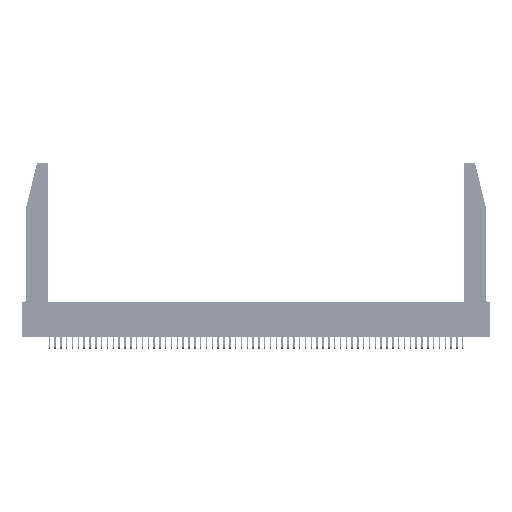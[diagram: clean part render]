
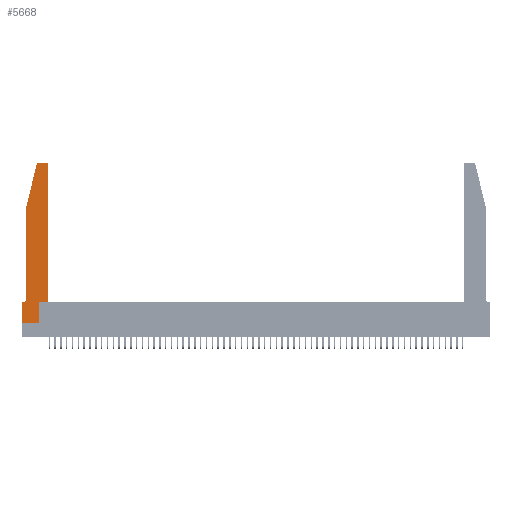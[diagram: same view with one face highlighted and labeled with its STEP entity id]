
A CAD part, top view. The second image highlights one B-rep face of the part: STEP entity #5668.
In plain terms, the highlighted planar face has unit normal (0, 0, 1).
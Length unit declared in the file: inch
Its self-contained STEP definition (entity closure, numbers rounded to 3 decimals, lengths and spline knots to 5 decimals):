
#886 = LINE ( 'NONE', #34064, #15802 ) ;
#995 = DIRECTION ( 'NONE',  ( 1., 0., 0. ) ) ;
#1114 = DIRECTION ( 'NONE',  ( 1., 0., 0. ) ) ;
#1176 = ORIENTED_EDGE ( 'NONE', *, *, #48175, .T. ) ;
#2003 = VECTOR ( 'NONE', #14188, 39.37008 ) ;
#2604 = AXIS2_PLACEMENT_3D ( 'NONE', #47285, #15888, #20061 ) ;
#2913 = CARTESIAN_POINT ( 'NONE',  ( 0.284, 2.75, 0.37 ) ) ;
#3391 = VERTEX_POINT ( 'NONE', #58541 ) ;
#3454 = VERTEX_POINT ( 'NONE', #50158 ) ;
#3979 = ORIENTED_EDGE ( 'NONE', *, *, #10739, .T. ) ;
#4267 = DIRECTION ( 'NONE',  ( 1., 0., 0. ) ) ;
#4681 = CARTESIAN_POINT ( 'NONE',  ( 0.2865, 0.35, 0.37 ) ) ;
#4703 = VERTEX_POINT ( 'NONE', #22399 ) ;
#5668 = ADVANCED_FACE ( 'NONE', ( #57663 ), #21222, .T. ) ;
#6243 = EDGE_CURVE ( 'NONE', #20756, #44122, #54789, .T. ) ;
#6296 = AXIS2_PLACEMENT_3D ( 'NONE', #31254, #8640, #4267 ) ;
#6351 = LINE ( 'NONE', #9696, #16989 ) ;
#6877 = LINE ( 'NONE', #51187, #18277 ) ;
#7014 = CARTESIAN_POINT ( 'NONE',  ( 0.4505, 0.35, 0.37 ) ) ;
#7945 = LINE ( 'NONE', #32631, #54228 ) ;
#8463 = DIRECTION ( 'NONE',  ( 0., -1., 0. ) ) ;
#8640 = DIRECTION ( 'NONE',  ( 0., 0., 1. ) ) ;
#8919 = CARTESIAN_POINT ( 'NONE',  ( 0.0755, 2., 0.37 ) ) ;
#9696 = CARTESIAN_POINT ( 'NONE',  ( 0.0755, 2., 0.37 ) ) ;
#9926 = ORIENTED_EDGE ( 'NONE', *, *, #46195, .T. ) ;
#10739 = EDGE_CURVE ( 'NONE', #12958, #4703, #27918, .T. ) ;
#12958 = VERTEX_POINT ( 'NONE', #2913 ) ;
#13223 = ORIENTED_EDGE ( 'NONE', *, *, #6243, .T. ) ;
#13413 = ORIENTED_EDGE ( 'NONE', *, *, #58193, .T. ) ;
#14188 = DIRECTION ( 'NONE',  ( -1., 0., 0. ) ) ;
#14907 = VERTEX_POINT ( 'NONE', #16679 ) ;
#15802 = VECTOR ( 'NONE', #38626, 39.37008 ) ;
#15888 = DIRECTION ( 'NONE',  ( 0., 0., 1. ) ) ;
#16183 = LINE ( 'NONE', #19146, #2003 ) ;
#16263 = DIRECTION ( 'NONE',  ( 1., 0., 0. ) ) ;
#16679 = CARTESIAN_POINT ( 'NONE',  ( 0., 0.35, 0.37 ) ) ;
#16792 = EDGE_CURVE ( 'NONE', #3391, #40836, #28212, .T. ) ;
#16989 = VECTOR ( 'NONE', #23176, 39.37008 ) ;
#17145 = CARTESIAN_POINT ( 'NONE',  ( 0.2865, 0., 0.37 ) ) ;
#18022 = ORIENTED_EDGE ( 'NONE', *, *, #32791, .T. ) ;
#18277 = VECTOR ( 'NONE', #1114, 39.37008 ) ;
#18356 = DIRECTION ( 'NONE',  ( 0., 1., 0. ) ) ;
#19067 = VECTOR ( 'NONE', #8463, 39.37008 ) ;
#19146 = CARTESIAN_POINT ( 'NONE',  ( 0.2605, 2.75, 0.37 ) ) ;
#20061 = DIRECTION ( 'NONE',  ( 1., 0., 0. ) ) ;
#20134 = ORIENTED_EDGE ( 'NONE', *, *, #22458, .T. ) ;
#20735 = CARTESIAN_POINT ( 'NONE',  ( 0.2865, 0.35, 0.37 ) ) ;
#20743 = LINE ( 'NONE', #4681, #44160 ) ;
#20756 = VERTEX_POINT ( 'NONE', #44399 ) ;
#21025 = CARTESIAN_POINT ( 'NONE',  ( 0.0055, 0.35, 0.37 ) ) ;
#21222 = PLANE ( 'NONE',  #37858 ) ;
#22399 = CARTESIAN_POINT ( 'NONE',  ( 0.25487, 2.72718, 0.37 ) ) ;
#22458 = EDGE_CURVE ( 'NONE', #14907, #3391, #51081, .T. ) ;
#23133 = CIRCLE ( 'NONE', #6296, 0.03 ) ;
#23176 = DIRECTION ( 'NONE',  ( -0.239, -0.971, 0. ) ) ;
#23541 = DIRECTION ( 'NONE',  ( -1., 0., 0. ) ) ;
#23773 = VERTEX_POINT ( 'NONE', #7014 ) ;
#26167 = CARTESIAN_POINT ( 'NONE',  ( 0., 0.35, 0.37 ) ) ;
#26787 = VECTOR ( 'NONE', #995, 39.37008 ) ;
#27918 = CIRCLE ( 'NONE', #2604, 0.03 ) ;
#28001 = ORIENTED_EDGE ( 'NONE', *, *, #55829, .T. ) ;
#28212 = LINE ( 'NONE', #55469, #26787 ) ;
#28951 = EDGE_LOOP ( 'NONE', ( #1176, #3979, #44353, #44969, #13223, #28001, #20134, #52502, #9926, #13413, #39489, #18022 ) ) ;
#30172 = CARTESIAN_POINT ( 'NONE',  ( 0.0755, 0.35, 0.37 ) ) ;
#31254 = CARTESIAN_POINT ( 'NONE',  ( 0.4205, 2.72, 0.37 ) ) ;
#32631 = CARTESIAN_POINT ( 'NONE',  ( 0.0755, 2., 0.37 ) ) ;
#32791 = EDGE_CURVE ( 'NONE', #54152, #3454, #23133, .T. ) ;
#34064 = CARTESIAN_POINT ( 'NONE',  ( 0.4505, 0.35, 0.37 ) ) ;
#35205 = EDGE_CURVE ( 'NONE', #23773, #54152, #886, .T. ) ;
#35310 = DIRECTION ( 'NONE',  ( 0., 0., 1. ) ) ;
#36758 = VERTEX_POINT ( 'NONE', #8919 ) ;
#36897 = EDGE_CURVE ( 'NONE', #4703, #36758, #6351, .T. ) ;
#37858 = AXIS2_PLACEMENT_3D ( 'NONE', #26167, #35310, #16263 ) ;
#38626 = DIRECTION ( 'NONE',  ( 0., 1., 0. ) ) ;
#39489 = ORIENTED_EDGE ( 'NONE', *, *, #35205, .T. ) ;
#40836 = VERTEX_POINT ( 'NONE', #17145 ) ;
#41428 = CARTESIAN_POINT ( 'NONE',  ( 0.0055, 0.42, 0.37 ) ) ;
#44122 = VERTEX_POINT ( 'NONE', #21025 ) ;
#44160 = VECTOR ( 'NONE', #18356, 39.37008 ) ;
#44353 = ORIENTED_EDGE ( 'NONE', *, *, #36897, .T. ) ;
#44399 = CARTESIAN_POINT ( 'NONE',  ( 0.0755, 0.42, 0.37 ) ) ;
#44851 = LINE ( 'NONE', #30172, #51269 ) ;
#44969 = ORIENTED_EDGE ( 'NONE', *, *, #46278, .T. ) ;
#45078 = AXIS2_PLACEMENT_3D ( 'NONE', #41428, #50798, #23541 ) ;
#46195 = EDGE_CURVE ( 'NONE', #40836, #58361, #20743, .T. ) ;
#46278 = EDGE_CURVE ( 'NONE', #36758, #20756, #7945, .T. ) ;
#46736 = DIRECTION ( 'NONE',  ( 0., -1., 0. ) ) ;
#47285 = CARTESIAN_POINT ( 'NONE',  ( 0.284, 2.72, 0.37 ) ) ;
#47689 = DIRECTION ( 'NONE',  ( -1., 0., 0. ) ) ;
#48175 = EDGE_CURVE ( 'NONE', #3454, #12958, #16183, .T. ) ;
#50158 = CARTESIAN_POINT ( 'NONE',  ( 0.4205, 2.75, 0.37 ) ) ;
#50798 = DIRECTION ( 'NONE',  ( 0., 0., -1. ) ) ;
#51081 = LINE ( 'NONE', #57763, #19067 ) ;
#51187 = CARTESIAN_POINT ( 'NONE',  ( 0.4505, 0.35, 0.37 ) ) ;
#51269 = VECTOR ( 'NONE', #47689, 39.37008 ) ;
#52502 = ORIENTED_EDGE ( 'NONE', *, *, #16792, .T. ) ;
#54152 = VERTEX_POINT ( 'NONE', #56172 ) ;
#54228 = VECTOR ( 'NONE', #46736, 39.37008 ) ;
#54789 = CIRCLE ( 'NONE', #45078, 0.07 ) ;
#55469 = CARTESIAN_POINT ( 'NONE',  ( 0., 0., 0.37 ) ) ;
#55829 = EDGE_CURVE ( 'NONE', #44122, #14907, #44851, .T. ) ;
#56172 = CARTESIAN_POINT ( 'NONE',  ( 0.4505, 2.72, 0.37 ) ) ;
#57663 = FACE_OUTER_BOUND ( 'NONE', #28951, .T. ) ;
#57763 = CARTESIAN_POINT ( 'NONE',  ( 0., 0., 0.37 ) ) ;
#58193 = EDGE_CURVE ( 'NONE', #58361, #23773, #6877, .T. ) ;
#58361 = VERTEX_POINT ( 'NONE', #20735 ) ;
#58541 = CARTESIAN_POINT ( 'NONE',  ( 0., 0., 0.37 ) ) ;
